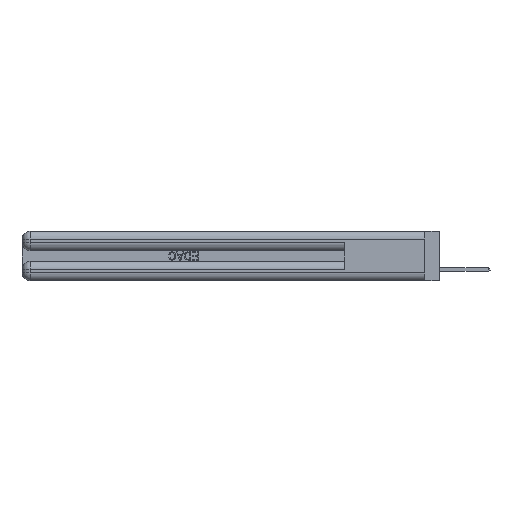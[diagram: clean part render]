
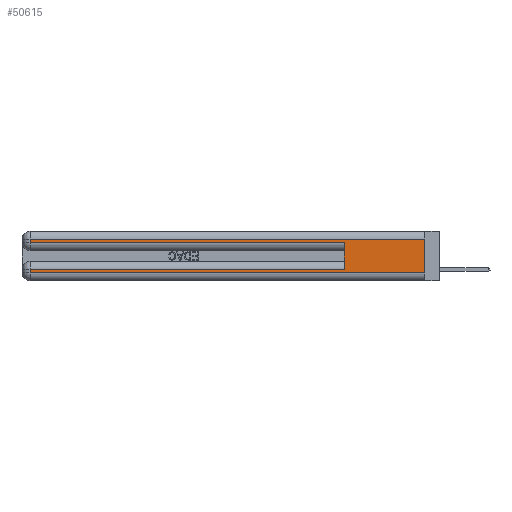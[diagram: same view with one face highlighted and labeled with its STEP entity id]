
A CAD part, left-side view. The second image highlights one B-rep face of the part: STEP entity #50615.
In plain terms, the highlighted planar face has unit normal (-1, 0, 0).
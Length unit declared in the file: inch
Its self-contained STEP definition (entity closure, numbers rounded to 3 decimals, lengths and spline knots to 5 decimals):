
#1070 = CARTESIAN_POINT ( 'NONE',  ( 0., 0., 0.31 ) ) ;
#2063 = ORIENTED_EDGE ( 'NONE', *, *, #36970, .T. ) ;
#3672 = VECTOR ( 'NONE', #22267, 39.37008 ) ;
#3674 = CARTESIAN_POINT ( 'NONE',  ( 0., 0., 0.06 ) ) ;
#5485 = DIRECTION ( 'NONE',  ( 0., 0., -1. ) ) ;
#9250 = VERTEX_POINT ( 'NONE', #10442 ) ;
#9677 = VECTOR ( 'NONE', #29611, 39.37008 ) ;
#10233 = LINE ( 'NONE', #27672, #18594 ) ;
#10442 = CARTESIAN_POINT ( 'NONE',  ( 0., 0.6, 0.285 ) ) ;
#10448 = CARTESIAN_POINT ( 'NONE',  ( 0., 2.94, 0.37 ) ) ;
#12008 = VERTEX_POINT ( 'NONE', #1070 ) ;
#12011 = ORIENTED_EDGE ( 'NONE', *, *, #18619, .T. ) ;
#12205 = AXIS2_PLACEMENT_3D ( 'NONE', #37737, #29837, #5485 ) ;
#12862 = ORIENTED_EDGE ( 'NONE', *, *, #35800, .F. ) ;
#13124 = CARTESIAN_POINT ( 'NONE',  ( 0., 0., 0.085 ) ) ;
#13257 = VECTOR ( 'NONE', #48597, 39.37008 ) ;
#13484 = CARTESIAN_POINT ( 'NONE',  ( 0., 0., 0.06 ) ) ;
#14854 = EDGE_CURVE ( 'NONE', #43203, #35355, #35357, .T. ) ;
#16011 = CARTESIAN_POINT ( 'NONE',  ( 0., 2.94, 0.085 ) ) ;
#16412 = LINE ( 'NONE', #10448, #3672 ) ;
#16879 = CARTESIAN_POINT ( 'NONE',  ( 0., 0., 0.37 ) ) ;
#18594 = VECTOR ( 'NONE', #35349, 39.37008 ) ;
#18619 = EDGE_CURVE ( 'NONE', #35355, #36433, #16412, .T. ) ;
#19260 = DIRECTION ( 'NONE',  ( 0., 0., 1. ) ) ;
#20978 = ORIENTED_EDGE ( 'NONE', *, *, #49858, .T. ) ;
#21207 = DIRECTION ( 'NONE',  ( 0., 1., 0. ) ) ;
#21367 = EDGE_CURVE ( 'NONE', #12008, #29306, #28168, .T. ) ;
#22142 = EDGE_CURVE ( 'NONE', #31662, #9250, #36355, .T. ) ;
#22267 = DIRECTION ( 'NONE',  ( 0., 0., -1. ) ) ;
#22776 = CARTESIAN_POINT ( 'NONE',  ( 0., 2.94, 0.285 ) ) ;
#22814 = DIRECTION ( 'NONE',  ( 0., -1., 0. ) ) ;
#23007 = VECTOR ( 'NONE', #21207, 39.37008 ) ;
#24027 = LINE ( 'NONE', #16879, #52222 ) ;
#24240 = LINE ( 'NONE', #3674, #13257 ) ;
#25431 = VECTOR ( 'NONE', #22814, 39.37008 ) ;
#25637 = DIRECTION ( 'NONE',  ( 0., 0., -1. ) ) ;
#26567 = CARTESIAN_POINT ( 'NONE',  ( 0., 0., 0.285 ) ) ;
#26804 = CARTESIAN_POINT ( 'NONE',  ( 0., 0.6, 0.085 ) ) ;
#27672 = CARTESIAN_POINT ( 'NONE',  ( 0., 2.94, 0.37 ) ) ;
#28168 = LINE ( 'NONE', #33954, #23007 ) ;
#28935 = LINE ( 'NONE', #34442, #31564 ) ;
#29013 = EDGE_LOOP ( 'NONE', ( #33287, #47497, #2063, #31708, #12862, #34331, #12011, #20978 ) ) ;
#29306 = VERTEX_POINT ( 'NONE', #41066 ) ;
#29611 = DIRECTION ( 'NONE',  ( 0., 1., 0. ) ) ;
#29837 = DIRECTION ( 'NONE',  ( 1., 0., 0. ) ) ;
#31564 = VECTOR ( 'NONE', #19260, 39.37008 ) ;
#31662 = VERTEX_POINT ( 'NONE', #22776 ) ;
#31708 = ORIENTED_EDGE ( 'NONE', *, *, #22142, .T. ) ;
#33287 = ORIENTED_EDGE ( 'NONE', *, *, #43638, .F. ) ;
#33954 = CARTESIAN_POINT ( 'NONE',  ( 0., 0., 0.31 ) ) ;
#34331 = ORIENTED_EDGE ( 'NONE', *, *, #14854, .T. ) ;
#34442 = CARTESIAN_POINT ( 'NONE',  ( 0., 0.6, 0.145 ) ) ;
#34674 = VERTEX_POINT ( 'NONE', #13484 ) ;
#35349 = DIRECTION ( 'NONE',  ( 0., 0., -1. ) ) ;
#35355 = VERTEX_POINT ( 'NONE', #16011 ) ;
#35357 = LINE ( 'NONE', #13124, #9677 ) ;
#35603 = FACE_OUTER_BOUND ( 'NONE', #29013, .T. ) ;
#35800 = EDGE_CURVE ( 'NONE', #43203, #9250, #28935, .T. ) ;
#36355 = LINE ( 'NONE', #26567, #25431 ) ;
#36433 = VERTEX_POINT ( 'NONE', #37837 ) ;
#36970 = EDGE_CURVE ( 'NONE', #29306, #31662, #10233, .T. ) ;
#37737 = CARTESIAN_POINT ( 'NONE',  ( 0., 0., 0.37 ) ) ;
#37837 = CARTESIAN_POINT ( 'NONE',  ( 0., 2.94, 0.06 ) ) ;
#41066 = CARTESIAN_POINT ( 'NONE',  ( 0., 2.94, 0.31 ) ) ;
#43203 = VERTEX_POINT ( 'NONE', #26804 ) ;
#43638 = EDGE_CURVE ( 'NONE', #12008, #34674, #24027, .T. ) ;
#47497 = ORIENTED_EDGE ( 'NONE', *, *, #21367, .T. ) ;
#48597 = DIRECTION ( 'NONE',  ( 0., -1., 0. ) ) ;
#49858 = EDGE_CURVE ( 'NONE', #36433, #34674, #24240, .T. ) ;
#49880 = PLANE ( 'NONE',  #12205 ) ;
#50615 = ADVANCED_FACE ( 'NONE', ( #35603 ), #49880, .F. ) ;
#52222 = VECTOR ( 'NONE', #25637, 39.37008 ) ;
